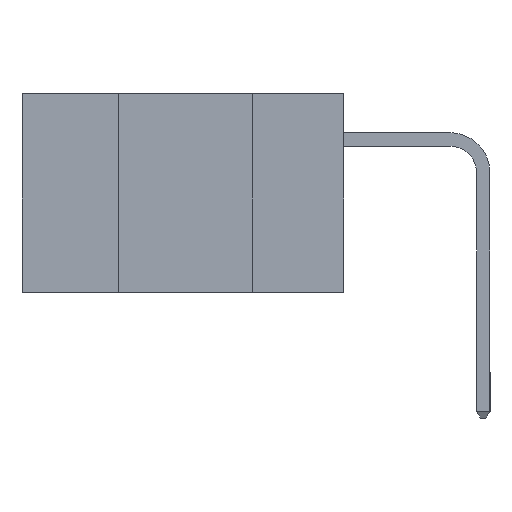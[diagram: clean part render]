
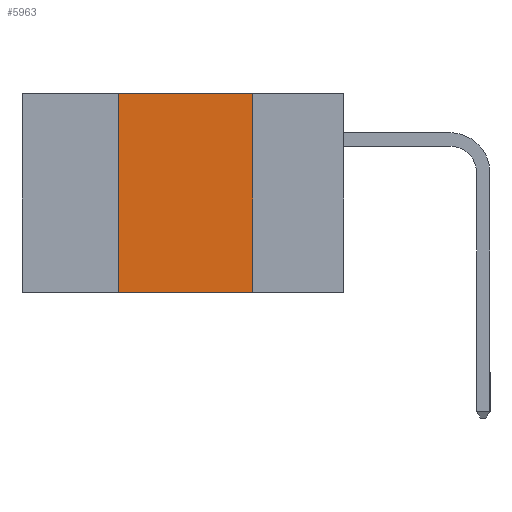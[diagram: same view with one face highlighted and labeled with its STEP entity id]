
A CAD part, left-side view. The second image highlights one B-rep face of the part: STEP entity #5963.
In plain terms, the highlighted planar face has unit normal (-1, 0, 0).
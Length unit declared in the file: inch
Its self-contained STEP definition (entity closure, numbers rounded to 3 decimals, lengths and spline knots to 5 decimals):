
#356 = VECTOR ( 'NONE', #9858, 39.37008 ) ;
#454 = VECTOR ( 'NONE', #11336, 39.37008 ) ;
#528 = EDGE_CURVE ( 'NONE', #10088, #5918, #10807, .T. ) ;
#826 = CARTESIAN_POINT ( 'NONE',  ( 0., 0.6, 0. ) ) ;
#967 = CARTESIAN_POINT ( 'NONE',  ( 0., 0.6, -0.37 ) ) ;
#998 = ORIENTED_EDGE ( 'NONE', *, *, #6114, .F. ) ;
#1340 = CARTESIAN_POINT ( 'NONE',  ( 0., 0.42, -0.37 ) ) ;
#1489 = DIRECTION ( 'NONE',  ( 0., -1., 0. ) ) ;
#2366 = EDGE_CURVE ( 'NONE', #5825, #5918, #5475, .T. ) ;
#2663 = ORIENTED_EDGE ( 'NONE', *, *, #2366, .F. ) ;
#3508 = CARTESIAN_POINT ( 'NONE',  ( 0., 0.42, 0. ) ) ;
#4024 = CARTESIAN_POINT ( 'NONE',  ( 0., 0.17, 0. ) ) ;
#4074 = FACE_OUTER_BOUND ( 'NONE', #7681, .T. ) ;
#4103 = AXIS2_PLACEMENT_3D ( 'NONE', #826, #7175, #7254 ) ;
#4579 = VERTEX_POINT ( 'NONE', #3508 ) ;
#4869 = CARTESIAN_POINT ( 'NONE',  ( 0., 0.42, 0. ) ) ;
#5475 = LINE ( 'NONE', #8995, #356 ) ;
#5825 = VERTEX_POINT ( 'NONE', #4024 ) ;
#5918 = VERTEX_POINT ( 'NONE', #7961 ) ;
#5963 = ADVANCED_FACE ( 'NONE', ( #4074 ), #7215, .F. ) ;
#6114 = EDGE_CURVE ( 'NONE', #4579, #5825, #10342, .T. ) ;
#7119 = LINE ( 'NONE', #4869, #454 ) ;
#7175 = DIRECTION ( 'NONE',  ( 1., 0., 0. ) ) ;
#7215 = PLANE ( 'NONE',  #4103 ) ;
#7254 = DIRECTION ( 'NONE',  ( 0., 0., -1. ) ) ;
#7411 = DIRECTION ( 'NONE',  ( 0., -1., 0. ) ) ;
#7681 = EDGE_LOOP ( 'NONE', ( #2663, #998, #11295, #10213 ) ) ;
#7961 = CARTESIAN_POINT ( 'NONE',  ( 0., 0.17, -0.37 ) ) ;
#8995 = CARTESIAN_POINT ( 'NONE',  ( 0., 0.17, 0. ) ) ;
#9067 = EDGE_CURVE ( 'NONE', #10088, #4579, #7119, .T. ) ;
#9858 = DIRECTION ( 'NONE',  ( 0., 0., -1. ) ) ;
#10088 = VERTEX_POINT ( 'NONE', #1340 ) ;
#10213 = ORIENTED_EDGE ( 'NONE', *, *, #528, .T. ) ;
#10342 = LINE ( 'NONE', #10467, #10935 ) ;
#10467 = CARTESIAN_POINT ( 'NONE',  ( 0., 0.6, 0. ) ) ;
#10653 = VECTOR ( 'NONE', #7411, 39.37008 ) ;
#10807 = LINE ( 'NONE', #967, #10653 ) ;
#10935 = VECTOR ( 'NONE', #1489, 39.37008 ) ;
#11295 = ORIENTED_EDGE ( 'NONE', *, *, #9067, .F. ) ;
#11336 = DIRECTION ( 'NONE',  ( 0., 0., 1. ) ) ;
